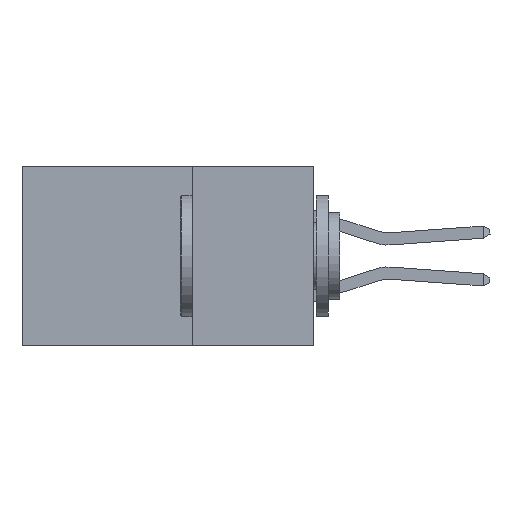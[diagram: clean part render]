
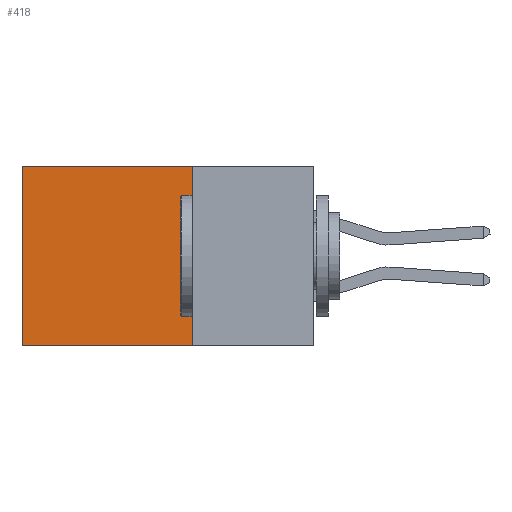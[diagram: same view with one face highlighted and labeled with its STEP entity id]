
A CAD part, left-side view. The second image highlights one B-rep face of the part: STEP entity #418.
In plain terms, the highlighted planar face has unit normal (-1, 0, 0).
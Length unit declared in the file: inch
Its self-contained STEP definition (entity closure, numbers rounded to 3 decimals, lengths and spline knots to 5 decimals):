
#238 = CARTESIAN_POINT ( 'NONE',  ( 0.2875, 0.25, -0.37 ) ) ;
#322 = CARTESIAN_POINT ( 'NONE',  ( 0.2875, 0.25, 0. ) ) ;
#374 = DIRECTION ( 'NONE',  ( 0., 0., -1. ) ) ;
#418 = ADVANCED_FACE ( 'NONE', ( #10807 ), #7401, .F. ) ;
#536 = EDGE_CURVE ( 'NONE', #13224, #7382, #3964, .T. ) ;
#762 = CARTESIAN_POINT ( 'NONE',  ( 0.2875, 0.25, -0.37 ) ) ;
#765 = LINE ( 'NONE', #11168, #6287 ) ;
#1584 = VERTEX_POINT ( 'NONE', #8566 ) ;
#2745 = VECTOR ( 'NONE', #374, 39.37008 ) ;
#2796 = EDGE_CURVE ( 'NONE', #1584, #13224, #6696, .T. ) ;
#2846 = ORIENTED_EDGE ( 'NONE', *, *, #8779, .T. ) ;
#2996 = DIRECTION ( 'NONE',  ( 0., 1., 0. ) ) ;
#3752 = VECTOR ( 'NONE', #7265, 39.37008 ) ;
#3964 = LINE ( 'NONE', #762, #5525 ) ;
#4060 = CARTESIAN_POINT ( 'NONE',  ( 0.2875, 0.25, 0. ) ) ;
#4099 = DIRECTION ( 'NONE',  ( 1., 0., 0. ) ) ;
#4142 = VERTEX_POINT ( 'NONE', #7918 ) ;
#4717 = CARTESIAN_POINT ( 'NONE',  ( 0.2875, 0.6, 0. ) ) ;
#5133 = DIRECTION ( 'NONE',  ( 0., 0., -1. ) ) ;
#5194 = EDGE_CURVE ( 'NONE', #1584, #4142, #765, .T. ) ;
#5525 = VECTOR ( 'NONE', #2996, 39.37008 ) ;
#6287 = VECTOR ( 'NONE', #6984, 39.37008 ) ;
#6696 = LINE ( 'NONE', #322, #3752 ) ;
#6984 = DIRECTION ( 'NONE',  ( 0., 1., 0. ) ) ;
#7265 = DIRECTION ( 'NONE',  ( 0., 0., -1. ) ) ;
#7382 = VERTEX_POINT ( 'NONE', #12302 ) ;
#7401 = PLANE ( 'NONE',  #8953 ) ;
#7610 = EDGE_LOOP ( 'NONE', ( #2846, #11278, #13817, #11511 ) ) ;
#7918 = CARTESIAN_POINT ( 'NONE',  ( 0.2875, 0.6, 0. ) ) ;
#8566 = CARTESIAN_POINT ( 'NONE',  ( 0.2875, 0.25, 0. ) ) ;
#8779 = EDGE_CURVE ( 'NONE', #4142, #7382, #10432, .T. ) ;
#8953 = AXIS2_PLACEMENT_3D ( 'NONE', #4060, #4099, #5133 ) ;
#10432 = LINE ( 'NONE', #4717, #2745 ) ;
#10807 = FACE_OUTER_BOUND ( 'NONE', #7610, .T. ) ;
#11168 = CARTESIAN_POINT ( 'NONE',  ( 0.2875, 0.25, 0. ) ) ;
#11278 = ORIENTED_EDGE ( 'NONE', *, *, #536, .F. ) ;
#11511 = ORIENTED_EDGE ( 'NONE', *, *, #5194, .T. ) ;
#12302 = CARTESIAN_POINT ( 'NONE',  ( 0.2875, 0.6, -0.37 ) ) ;
#13224 = VERTEX_POINT ( 'NONE', #238 ) ;
#13817 = ORIENTED_EDGE ( 'NONE', *, *, #2796, .F. ) ;
